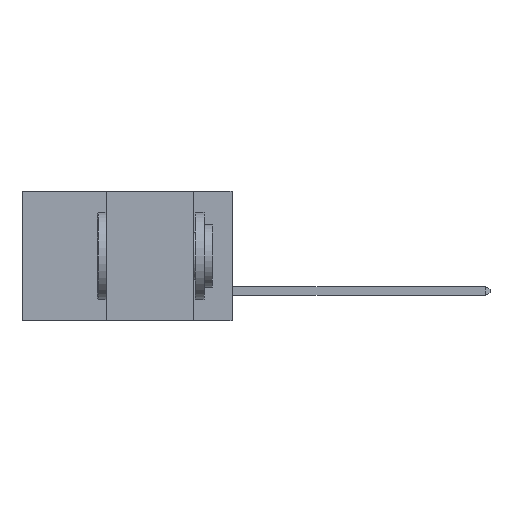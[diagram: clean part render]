
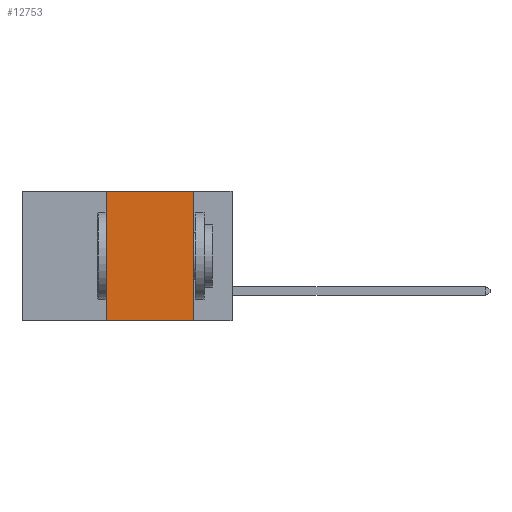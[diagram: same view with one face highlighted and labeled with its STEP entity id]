
A CAD part, left-side view. The second image highlights one B-rep face of the part: STEP entity #12753.
In plain terms, the highlighted planar face has unit normal (-1, 0, 0).
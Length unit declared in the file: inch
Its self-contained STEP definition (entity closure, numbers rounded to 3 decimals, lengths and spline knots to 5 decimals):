
#933 = ORIENTED_EDGE ( 'NONE', *, *, #2191, .F. ) ;
#1376 = DIRECTION ( 'NONE',  ( 0., 0., -1. ) ) ;
#1433 = CARTESIAN_POINT ( 'NONE',  ( 0., 0.11, 0. ) ) ;
#1550 = CARTESIAN_POINT ( 'NONE',  ( 0., 0.6, 0. ) ) ;
#1615 = VERTEX_POINT ( 'NONE', #18015 ) ;
#2001 = LINE ( 'NONE', #1433, #21473 ) ;
#2191 = EDGE_CURVE ( 'NONE', #1615, #7055, #2001, .T. ) ;
#2457 = EDGE_LOOP ( 'NONE', ( #933, #11139, #21598, #12355 ) ) ;
#2478 = CARTESIAN_POINT ( 'NONE',  ( 0., 0.6, -0.37 ) ) ;
#2955 = DIRECTION ( 'NONE',  ( 0., 0., 1. ) ) ;
#4022 = CARTESIAN_POINT ( 'NONE',  ( 0., 0.36, 0. ) ) ;
#5434 = VECTOR ( 'NONE', #12600, 39.37008 ) ;
#7055 = VERTEX_POINT ( 'NONE', #16412 ) ;
#7470 = PLANE ( 'NONE',  #21777 ) ;
#7673 = EDGE_CURVE ( 'NONE', #9411, #1615, #10476, .T. ) ;
#9175 = LINE ( 'NONE', #10672, #18468 ) ;
#9351 = DIRECTION ( 'NONE',  ( 0., 0., -1. ) ) ;
#9411 = VERTEX_POINT ( 'NONE', #4022 ) ;
#10216 = DIRECTION ( 'NONE',  ( 0., -1., 0. ) ) ;
#10476 = LINE ( 'NONE', #14382, #5434 ) ;
#10672 = CARTESIAN_POINT ( 'NONE',  ( 0., 0.36, 0. ) ) ;
#11139 = ORIENTED_EDGE ( 'NONE', *, *, #7673, .F. ) ;
#12326 = VECTOR ( 'NONE', #10216, 39.37008 ) ;
#12355 = ORIENTED_EDGE ( 'NONE', *, *, #15756, .T. ) ;
#12600 = DIRECTION ( 'NONE',  ( 0., -1., 0. ) ) ;
#12753 = ADVANCED_FACE ( 'NONE', ( #20803 ), #7470, .F. ) ;
#13744 = EDGE_CURVE ( 'NONE', #15207, #9411, #9175, .T. ) ;
#14382 = CARTESIAN_POINT ( 'NONE',  ( 0., 0.6, 0. ) ) ;
#15207 = VERTEX_POINT ( 'NONE', #23089 ) ;
#15756 = EDGE_CURVE ( 'NONE', #15207, #7055, #17844, .T. ) ;
#16412 = CARTESIAN_POINT ( 'NONE',  ( 0., 0.11, -0.37 ) ) ;
#17844 = LINE ( 'NONE', #2478, #12326 ) ;
#18015 = CARTESIAN_POINT ( 'NONE',  ( 0., 0.11, 0. ) ) ;
#18468 = VECTOR ( 'NONE', #2955, 39.37008 ) ;
#20445 = DIRECTION ( 'NONE',  ( 1., 0., 0. ) ) ;
#20803 = FACE_OUTER_BOUND ( 'NONE', #2457, .T. ) ;
#21473 = VECTOR ( 'NONE', #1376, 39.37008 ) ;
#21598 = ORIENTED_EDGE ( 'NONE', *, *, #13744, .F. ) ;
#21777 = AXIS2_PLACEMENT_3D ( 'NONE', #1550, #20445, #9351 ) ;
#23089 = CARTESIAN_POINT ( 'NONE',  ( 0., 0.36, -0.37 ) ) ;
